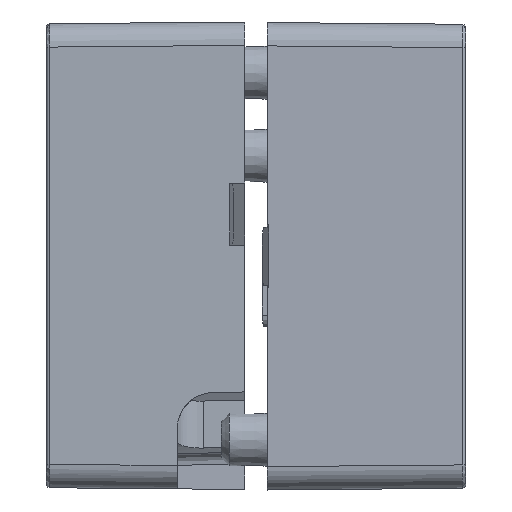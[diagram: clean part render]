
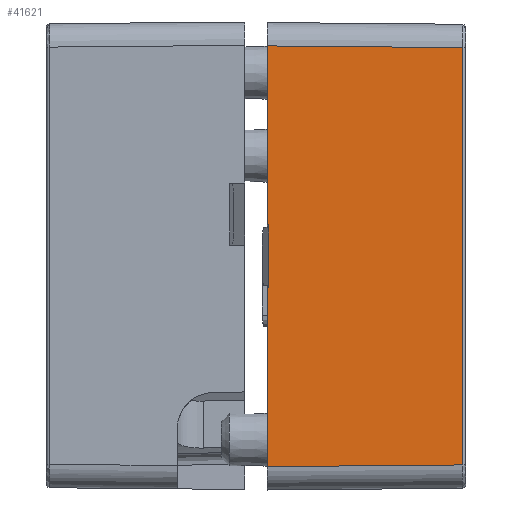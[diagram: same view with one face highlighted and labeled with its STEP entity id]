
A CAD part, left-side view. The second image highlights one B-rep face of the part: STEP entity #41621.
In plain terms, the highlighted planar face has unit normal (-1, -0.009, 0).
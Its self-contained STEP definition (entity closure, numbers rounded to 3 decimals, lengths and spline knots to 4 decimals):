
#4962=PLANE('',#44975);
#6724=FACE_OUTER_BOUND('',#9404,.T.);
#9404=EDGE_LOOP('',(#33967,#33968,#33969,#33970,#33971,#33972,#33973,#33974));
#12279=LINE('',#99943,#15134);
#12290=LINE('',#100075,#15145);
#12321=LINE('',#100693,#15176);
#12325=LINE('',#100764,#15180);
#12326=LINE('',#100766,#15181);
#12327=LINE('',#100768,#15182);
#12328=LINE('',#100769,#15183);
#12329=LINE('',#100770,#15184);
#15134=VECTOR('',#52329,1.);
#15145=VECTOR('',#52352,1.);
#15176=VECTOR('',#52475,1.);
#15180=VECTOR('',#52489,1.);
#15181=VECTOR('',#52490,1.);
#15182=VECTOR('',#52491,1.);
#15183=VECTOR('',#52492,1.);
#15184=VECTOR('',#52493,1.);
#18953=VERTEX_POINT('',#99940);
#18954=VERTEX_POINT('',#99942);
#18976=VERTEX_POINT('',#100072);
#18977=VERTEX_POINT('',#100074);
#19059=VERTEX_POINT('',#100685);
#19061=VERTEX_POINT('',#100691);
#19064=VERTEX_POINT('',#100765);
#19065=VERTEX_POINT('',#100767);
#24142=EDGE_CURVE('',#18953,#18954,#12279,.T.);
#24167=EDGE_CURVE('',#18976,#18977,#12290,.T.);
#24262=EDGE_CURVE('',#19061,#19059,#12321,.T.);
#24269=EDGE_CURVE('',#18977,#19061,#12325,.T.);
#24270=EDGE_CURVE('',#18976,#19064,#12326,.T.);
#24271=EDGE_CURVE('',#19064,#19065,#12327,.F.);
#24272=EDGE_CURVE('',#18954,#19065,#12328,.F.);
#24273=EDGE_CURVE('',#19059,#18953,#12329,.T.);
#33967=ORIENTED_EDGE('',*,*,#24262,.F.);
#33968=ORIENTED_EDGE('',*,*,#24269,.F.);
#33969=ORIENTED_EDGE('',*,*,#24167,.F.);
#33970=ORIENTED_EDGE('',*,*,#24270,.T.);
#33971=ORIENTED_EDGE('',*,*,#24271,.T.);
#33972=ORIENTED_EDGE('',*,*,#24272,.F.);
#33973=ORIENTED_EDGE('',*,*,#24142,.F.);
#33974=ORIENTED_EDGE('',*,*,#24273,.F.);
#41621=ADVANCED_FACE('',(#6724),#4962,.T.);
#44975=AXIS2_PLACEMENT_3D('',#100763,#52487,#52488);
#52329=DIRECTION('',(0.,0.,1.));
#52352=DIRECTION('',(0.,0.,1.));
#52475=DIRECTION('',(0.,0.,-1.));
#52487=DIRECTION('center_axis',(-1.,-0.009,
0.));
#52488=DIRECTION('ref_axis',(-0.009,1.,0.));
#52489=DIRECTION('',(0.009,-1.,-0.009));
#52490=DIRECTION('',(0.009,-1.,0.017));
#52491=DIRECTION('',(0.,0.,1.));
#52492=DIRECTION('',(-0.009,1.,0.017));
#52493=DIRECTION('',(-0.009,1.,-0.009));
#99940=CARTESIAN_POINT('',(-0.6567,0.,-2.1812));
#99942=CARTESIAN_POINT('',(-0.6567,0.,-1.415));
#99943=CARTESIAN_POINT('',(-0.6567,0.,-2.2892));
#100072=CARTESIAN_POINT('',(-0.6567,0.,-1.1472));
#100074=CARTESIAN_POINT('',(-0.6567,0.,-0.3812));
#100075=CARTESIAN_POINT('',(-0.6567,0.,-2.2892));
#100685=CARTESIAN_POINT('',(-0.6494,-0.8351,-2.1739));
#100691=CARTESIAN_POINT('',(-0.6494,-0.8351,-0.3884));
#100693=CARTESIAN_POINT('',(-0.6494,-0.8351,-0.9306));
#100763=CARTESIAN_POINT('Origin',(-0.6567,0.,-0.6446));
#100764=CARTESIAN_POINT('',(-0.6566,-0.0087,-0.3812));
#100765=CARTESIAN_POINT('',(-0.6566,-0.0062,-1.147));
#100766=CARTESIAN_POINT('',(-0.6566,-0.0048,-1.1471));
#100767=CARTESIAN_POINT('',(-0.6566,-0.0062,-1.4151));
#100768=CARTESIAN_POINT('',(-0.6566,-0.0062,-0.6426));
#100769=CARTESIAN_POINT('',(-0.6567,0.0057,-1.4149));
#100770=CARTESIAN_POINT('',(-0.6565,-0.0142,-2.181));
